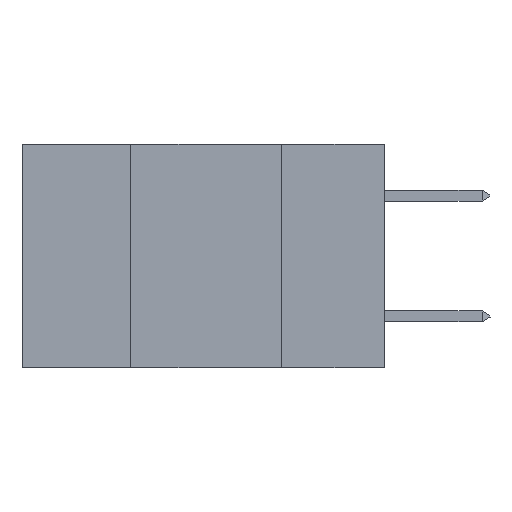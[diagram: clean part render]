
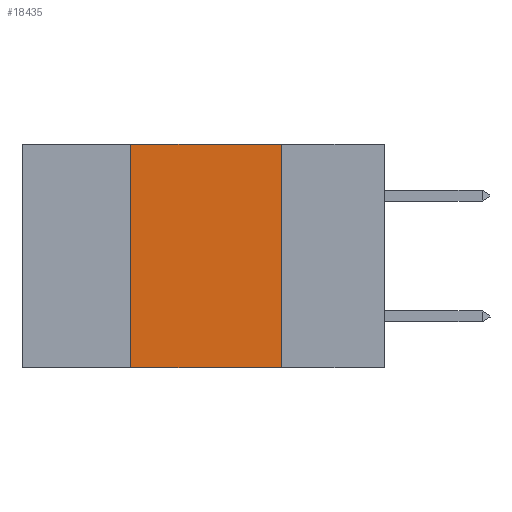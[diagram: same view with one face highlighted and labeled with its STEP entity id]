
A CAD part, left-side view. The second image highlights one B-rep face of the part: STEP entity #18435.
In plain terms, the highlighted planar face has unit normal (-1, 0, 0).
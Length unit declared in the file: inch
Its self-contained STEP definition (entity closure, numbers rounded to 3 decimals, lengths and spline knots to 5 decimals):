
#95 = EDGE_CURVE ( 'NONE', #11307, #19207, #797, .T. ) ;
#169 = EDGE_CURVE ( 'NONE', #18276, #18838, #14688, .T. ) ;
#797 = LINE ( 'NONE', #12903, #2590 ) ;
#1022 = ORIENTED_EDGE ( 'NONE', *, *, #95, .F. ) ;
#1354 = CARTESIAN_POINT ( 'NONE',  ( 0., 0.6, 0. ) ) ;
#2590 = VECTOR ( 'NONE', #16439, 39.37008 ) ;
#2619 = CARTESIAN_POINT ( 'NONE',  ( 0., 0.42, 0. ) ) ;
#2821 = AXIS2_PLACEMENT_3D ( 'NONE', #14168, #10976, #17427 ) ;
#3170 = DIRECTION ( 'NONE',  ( 0., -1., 0. ) ) ;
#4516 = LINE ( 'NONE', #1354, #7560 ) ;
#5059 = VECTOR ( 'NONE', #8213, 39.37008 ) ;
#5191 = ORIENTED_EDGE ( 'NONE', *, *, #9804, .T. ) ;
#5307 = ORIENTED_EDGE ( 'NONE', *, *, #17416, .F. ) ;
#5800 = CARTESIAN_POINT ( 'NONE',  ( 0., 0.42, -0.37 ) ) ;
#6798 = CARTESIAN_POINT ( 'NONE',  ( 0., 0.6, -0.37 ) ) ;
#6857 = VECTOR ( 'NONE', #14851, 39.37008 ) ;
#7560 = VECTOR ( 'NONE', #3170, 39.37008 ) ;
#7610 = PLANE ( 'NONE',  #2821 ) ;
#8213 = DIRECTION ( 'NONE',  ( 0., -1., 0. ) ) ;
#9541 = FACE_OUTER_BOUND ( 'NONE', #19519, .T. ) ;
#9614 = LINE ( 'NONE', #6798, #5059 ) ;
#9804 = EDGE_CURVE ( 'NONE', #18276, #19207, #9614, .T. ) ;
#10091 = CARTESIAN_POINT ( 'NONE',  ( 0., 0.42, 0. ) ) ;
#10976 = DIRECTION ( 'NONE',  ( 1., 0., 0. ) ) ;
#11307 = VERTEX_POINT ( 'NONE', #15368 ) ;
#12903 = CARTESIAN_POINT ( 'NONE',  ( 0., 0.17, 0. ) ) ;
#14168 = CARTESIAN_POINT ( 'NONE',  ( 0., 0.6, 0. ) ) ;
#14175 = CARTESIAN_POINT ( 'NONE',  ( 0., 0.17, -0.37 ) ) ;
#14688 = LINE ( 'NONE', #10091, #6857 ) ;
#14851 = DIRECTION ( 'NONE',  ( 0., 0., 1. ) ) ;
#15334 = ORIENTED_EDGE ( 'NONE', *, *, #169, .F. ) ;
#15368 = CARTESIAN_POINT ( 'NONE',  ( 0., 0.17, 0. ) ) ;
#16439 = DIRECTION ( 'NONE',  ( 0., 0., -1. ) ) ;
#17416 = EDGE_CURVE ( 'NONE', #18838, #11307, #4516, .T. ) ;
#17427 = DIRECTION ( 'NONE',  ( 0., 0., -1. ) ) ;
#18276 = VERTEX_POINT ( 'NONE', #5800 ) ;
#18435 = ADVANCED_FACE ( 'NONE', ( #9541 ), #7610, .F. ) ;
#18838 = VERTEX_POINT ( 'NONE', #2619 ) ;
#19207 = VERTEX_POINT ( 'NONE', #14175 ) ;
#19519 = EDGE_LOOP ( 'NONE', ( #1022, #5307, #15334, #5191 ) ) ;
